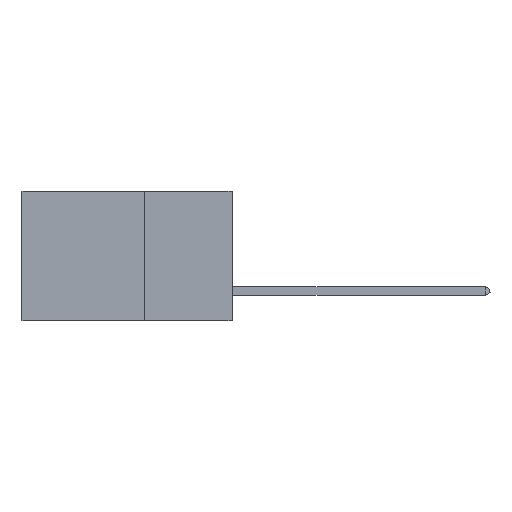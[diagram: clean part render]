
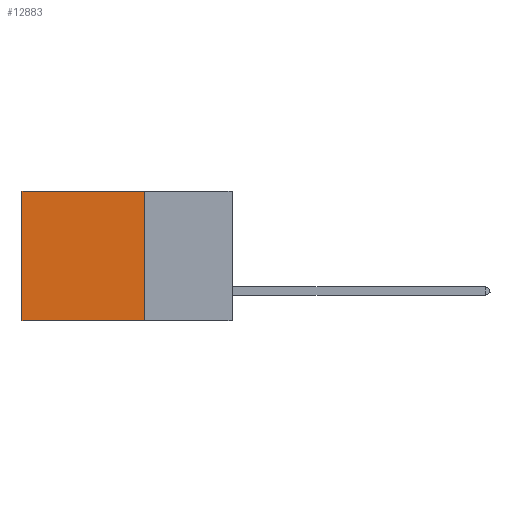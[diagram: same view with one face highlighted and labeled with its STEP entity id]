
A CAD part, left-side view. The second image highlights one B-rep face of the part: STEP entity #12883.
In plain terms, the highlighted planar face has unit normal (-1, 0, 0).
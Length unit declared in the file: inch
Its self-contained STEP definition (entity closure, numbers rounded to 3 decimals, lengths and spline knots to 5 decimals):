
#1092 = CARTESIAN_POINT ( 'NONE',  ( 0.2875, 0.6, -0.37 ) ) ;
#1431 = VECTOR ( 'NONE', #5185, 39.37008 ) ;
#2419 = CARTESIAN_POINT ( 'NONE',  ( 0.2875, 0.6, 0. ) ) ;
#4723 = DIRECTION ( 'NONE',  ( 0., 0., -1. ) ) ;
#5185 = DIRECTION ( 'NONE',  ( 0., 1., 0. ) ) ;
#6204 = CARTESIAN_POINT ( 'NONE',  ( 0.2875, 0.25, -0.37 ) ) ;
#7839 = ORIENTED_EDGE ( 'NONE', *, *, #14591, .F. ) ;
#8090 = VERTEX_POINT ( 'NONE', #1092 ) ;
#8877 = EDGE_CURVE ( 'NONE', #17915, #24666, #16070, .T. ) ;
#8887 = VECTOR ( 'NONE', #22158, 39.37008 ) ;
#9809 = LINE ( 'NONE', #23982, #8887 ) ;
#10294 = VECTOR ( 'NONE', #23933, 39.37008 ) ;
#10697 = FACE_OUTER_BOUND ( 'NONE', #19312, .T. ) ;
#11193 = ORIENTED_EDGE ( 'NONE', *, *, #22292, .F. ) ;
#11523 = CARTESIAN_POINT ( 'NONE',  ( 0.2875, 0.25, 0. ) ) ;
#12002 = CARTESIAN_POINT ( 'NONE',  ( 0.2875, 0.25, 0. ) ) ;
#12883 = ADVANCED_FACE ( 'NONE', ( #10697 ), #17892, .F. ) ;
#14591 = EDGE_CURVE ( 'NONE', #23131, #8090, #14927, .T. ) ;
#14927 = LINE ( 'NONE', #20925, #1431 ) ;
#15643 = DIRECTION ( 'NONE',  ( 0., 1., 0. ) ) ;
#15797 = ORIENTED_EDGE ( 'NONE', *, *, #8877, .T. ) ;
#15802 = CARTESIAN_POINT ( 'NONE',  ( 0.2875, 0.25, 0. ) ) ;
#16070 = LINE ( 'NONE', #15802, #22870 ) ;
#17482 = AXIS2_PLACEMENT_3D ( 'NONE', #12002, #22461, #4723 ) ;
#17892 = PLANE ( 'NONE',  #17482 ) ;
#17915 = VERTEX_POINT ( 'NONE', #11523 ) ;
#18503 = CARTESIAN_POINT ( 'NONE',  ( 0.2875, 0.6, 0. ) ) ;
#19172 = EDGE_CURVE ( 'NONE', #24666, #8090, #24189, .T. ) ;
#19312 = EDGE_LOOP ( 'NONE', ( #20162, #7839, #11193, #15797 ) ) ;
#20162 = ORIENTED_EDGE ( 'NONE', *, *, #19172, .T. ) ;
#20925 = CARTESIAN_POINT ( 'NONE',  ( 0.2875, 0.25, -0.37 ) ) ;
#22158 = DIRECTION ( 'NONE',  ( 0., 0., -1. ) ) ;
#22292 = EDGE_CURVE ( 'NONE', #17915, #23131, #9809, .T. ) ;
#22461 = DIRECTION ( 'NONE',  ( 1., 0., 0. ) ) ;
#22870 = VECTOR ( 'NONE', #15643, 39.37008 ) ;
#23131 = VERTEX_POINT ( 'NONE', #6204 ) ;
#23933 = DIRECTION ( 'NONE',  ( 0., 0., -1. ) ) ;
#23982 = CARTESIAN_POINT ( 'NONE',  ( 0.2875, 0.25, 0. ) ) ;
#24189 = LINE ( 'NONE', #2419, #10294 ) ;
#24666 = VERTEX_POINT ( 'NONE', #18503 ) ;
